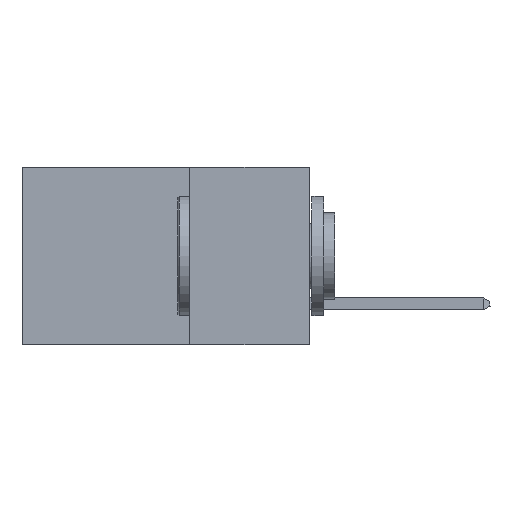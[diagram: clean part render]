
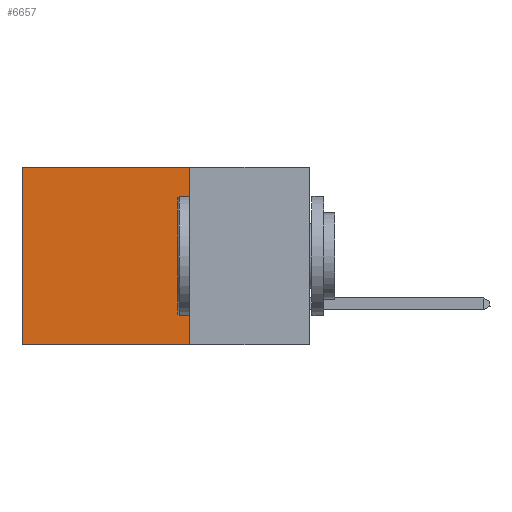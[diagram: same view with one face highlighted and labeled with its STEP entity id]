
A CAD part, left-side view. The second image highlights one B-rep face of the part: STEP entity #6657.
In plain terms, the highlighted planar face has unit normal (-1, 0, 0).
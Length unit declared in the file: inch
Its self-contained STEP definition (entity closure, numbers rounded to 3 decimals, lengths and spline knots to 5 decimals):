
#272 = EDGE_CURVE ( 'NONE', #16570, #5920, #10561, .T. ) ;
#297 = VECTOR ( 'NONE', #3500, 39.37008 ) ;
#458 = CARTESIAN_POINT ( 'NONE',  ( 0.2875, 0.25, 0. ) ) ;
#1390 = LINE ( 'NONE', #17341, #297 ) ;
#3500 = DIRECTION ( 'NONE',  ( 0., 0., -1. ) ) ;
#4392 = CARTESIAN_POINT ( 'NONE',  ( 0.2875, 0.25, -0.37 ) ) ;
#4394 = EDGE_CURVE ( 'NONE', #13385, #11282, #22207, .T. ) ;
#4529 = ORIENTED_EDGE ( 'NONE', *, *, #4394, .F. ) ;
#5354 = EDGE_CURVE ( 'NONE', #5920, #11282, #13312, .T. ) ;
#5499 = CARTESIAN_POINT ( 'NONE',  ( 0.2875, 0.6, 0. ) ) ;
#5920 = VERTEX_POINT ( 'NONE', #5499 ) ;
#6355 = DIRECTION ( 'NONE',  ( 0., 1., 0. ) ) ;
#6657 = ADVANCED_FACE ( 'NONE', ( #21821 ), #17979, .F. ) ;
#7559 = CARTESIAN_POINT ( 'NONE',  ( 0.2875, 0.25, 0. ) ) ;
#9340 = DIRECTION ( 'NONE',  ( 1., 0., 0. ) ) ;
#9687 = ORIENTED_EDGE ( 'NONE', *, *, #272, .T. ) ;
#10561 = LINE ( 'NONE', #10959, #15157 ) ;
#10571 = ORIENTED_EDGE ( 'NONE', *, *, #5354, .T. ) ;
#10867 = DIRECTION ( 'NONE',  ( 0., 0., -1. ) ) ;
#10959 = CARTESIAN_POINT ( 'NONE',  ( 0.2875, 0.25, 0. ) ) ;
#11127 = ORIENTED_EDGE ( 'NONE', *, *, #22198, .F. ) ;
#11282 = VERTEX_POINT ( 'NONE', #16045 ) ;
#13312 = LINE ( 'NONE', #14341, #22412 ) ;
#13385 = VERTEX_POINT ( 'NONE', #4392 ) ;
#13632 = VECTOR ( 'NONE', #6355, 39.37008 ) ;
#14341 = CARTESIAN_POINT ( 'NONE',  ( 0.2875, 0.6, 0. ) ) ;
#15157 = VECTOR ( 'NONE', #17731, 39.37008 ) ;
#16045 = CARTESIAN_POINT ( 'NONE',  ( 0.2875, 0.6, -0.37 ) ) ;
#16570 = VERTEX_POINT ( 'NONE', #458 ) ;
#17341 = CARTESIAN_POINT ( 'NONE',  ( 0.2875, 0.25, 0. ) ) ;
#17731 = DIRECTION ( 'NONE',  ( 0., 1., 0. ) ) ;
#17979 = PLANE ( 'NONE',  #22285 ) ;
#18509 = CARTESIAN_POINT ( 'NONE',  ( 0.2875, 0.25, -0.37 ) ) ;
#21392 = DIRECTION ( 'NONE',  ( 0., 0., -1. ) ) ;
#21790 = EDGE_LOOP ( 'NONE', ( #10571, #4529, #11127, #9687 ) ) ;
#21821 = FACE_OUTER_BOUND ( 'NONE', #21790, .T. ) ;
#22198 = EDGE_CURVE ( 'NONE', #16570, #13385, #1390, .T. ) ;
#22207 = LINE ( 'NONE', #18509, #13632 ) ;
#22285 = AXIS2_PLACEMENT_3D ( 'NONE', #7559, #9340, #21392 ) ;
#22412 = VECTOR ( 'NONE', #10867, 39.37008 ) ;
